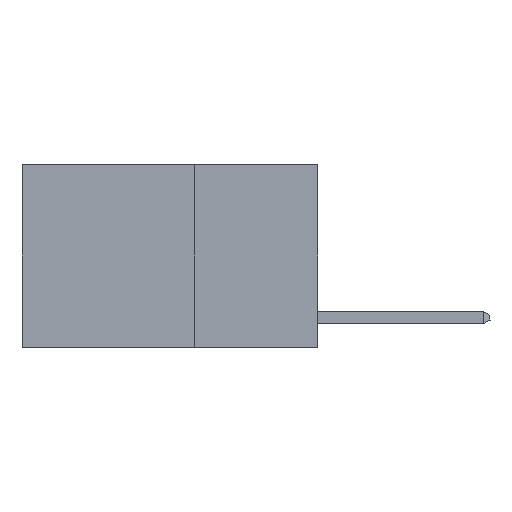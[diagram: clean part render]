
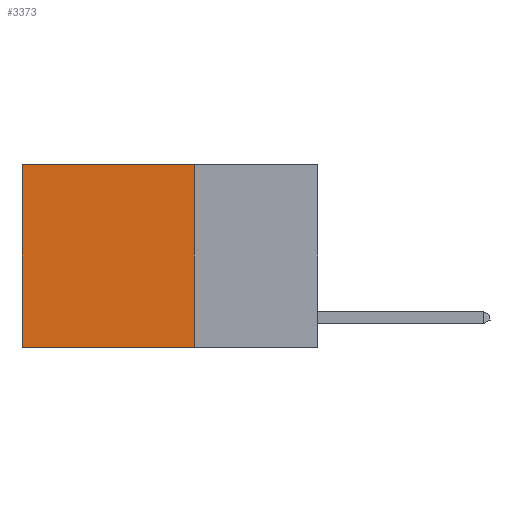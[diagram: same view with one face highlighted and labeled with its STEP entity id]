
A CAD part, left-side view. The second image highlights one B-rep face of the part: STEP entity #3373.
In plain terms, the highlighted planar face has unit normal (-1, 0, 0).
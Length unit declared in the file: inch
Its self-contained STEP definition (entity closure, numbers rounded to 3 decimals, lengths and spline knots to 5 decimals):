
#47 = CARTESIAN_POINT ( 'NONE',  ( 0.2625, 0.6, -0.37 ) ) ;
#2854 = LINE ( 'NONE', #20526, #23640 ) ;
#3215 = DIRECTION ( 'NONE',  ( 0., 0., -1. ) ) ;
#3373 = ADVANCED_FACE ( 'NONE', ( #17691 ), #9315, .F. ) ;
#4735 = ORIENTED_EDGE ( 'NONE', *, *, #22599, .T. ) ;
#5686 = DIRECTION ( 'NONE',  ( 0., 1., 0. ) ) ;
#6311 = CARTESIAN_POINT ( 'NONE',  ( 0.2625, 0.6, 0. ) ) ;
#7229 = LINE ( 'NONE', #21409, #22597 ) ;
#7452 = EDGE_CURVE ( 'NONE', #18872, #16034, #21243, .T. ) ;
#8435 = LINE ( 'NONE', #17742, #25030 ) ;
#8740 = CARTESIAN_POINT ( 'NONE',  ( 0.2625, 0.25, 0. ) ) ;
#9315 = PLANE ( 'NONE',  #21488 ) ;
#13043 = ORIENTED_EDGE ( 'NONE', *, *, #25802, .T. ) ;
#13317 = CARTESIAN_POINT ( 'NONE',  ( 0.2625, 0.25, 0. ) ) ;
#14075 = EDGE_LOOP ( 'NONE', ( #4735, #16128, #21940, #13043 ) ) ;
#15332 = DIRECTION ( 'NONE',  ( 1., 0., 0. ) ) ;
#16034 = VERTEX_POINT ( 'NONE', #23301 ) ;
#16128 = ORIENTED_EDGE ( 'NONE', *, *, #20431, .F. ) ;
#17691 = FACE_OUTER_BOUND ( 'NONE', #14075, .T. ) ;
#17742 = CARTESIAN_POINT ( 'NONE',  ( 0.2625, 0.25, 0. ) ) ;
#18872 = VERTEX_POINT ( 'NONE', #8740 ) ;
#19573 = CARTESIAN_POINT ( 'NONE',  ( 0.2625, 0.25, 0. ) ) ;
#20431 = EDGE_CURVE ( 'NONE', #16034, #23112, #7229, .T. ) ;
#20526 = CARTESIAN_POINT ( 'NONE',  ( 0.2625, 0.6, 0. ) ) ;
#21243 = LINE ( 'NONE', #19573, #25954 ) ;
#21409 = CARTESIAN_POINT ( 'NONE',  ( 0.2625, 0.25, -0.37 ) ) ;
#21488 = AXIS2_PLACEMENT_3D ( 'NONE', #13317, #15332, #3215 ) ;
#21940 = ORIENTED_EDGE ( 'NONE', *, *, #7452, .F. ) ;
#22597 = VECTOR ( 'NONE', #23409, 39.37008 ) ;
#22599 = EDGE_CURVE ( 'NONE', #24176, #23112, #2854, .T. ) ;
#23112 = VERTEX_POINT ( 'NONE', #47 ) ;
#23301 = CARTESIAN_POINT ( 'NONE',  ( 0.2625, 0.25, -0.37 ) ) ;
#23409 = DIRECTION ( 'NONE',  ( 0., 1., 0. ) ) ;
#23472 = DIRECTION ( 'NONE',  ( 0., 0., -1. ) ) ;
#23640 = VECTOR ( 'NONE', #24535, 39.37008 ) ;
#24176 = VERTEX_POINT ( 'NONE', #6311 ) ;
#24535 = DIRECTION ( 'NONE',  ( 0., 0., -1. ) ) ;
#25030 = VECTOR ( 'NONE', #5686, 39.37008 ) ;
#25802 = EDGE_CURVE ( 'NONE', #18872, #24176, #8435, .T. ) ;
#25954 = VECTOR ( 'NONE', #23472, 39.37008 ) ;
